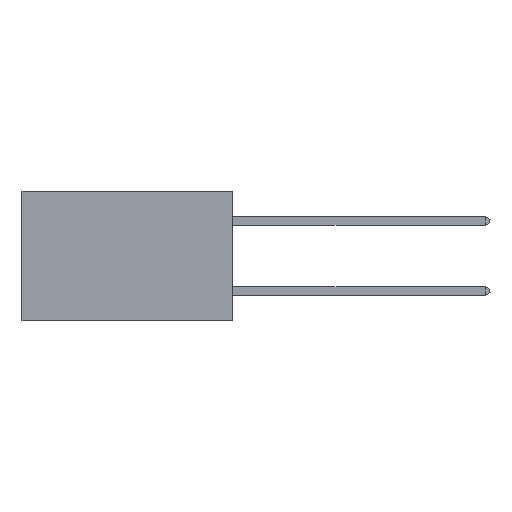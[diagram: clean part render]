
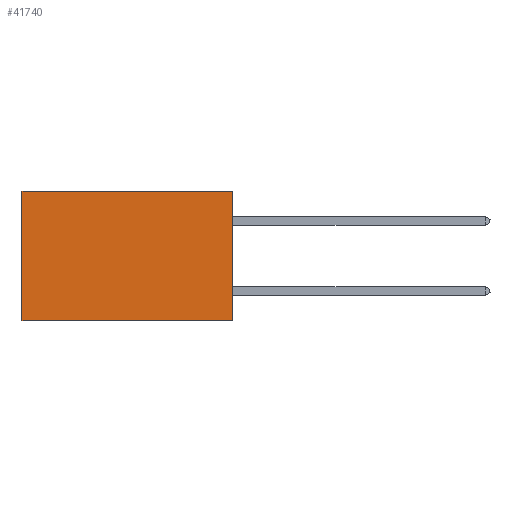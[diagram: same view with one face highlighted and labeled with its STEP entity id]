
A CAD part, left-side view. The second image highlights one B-rep face of the part: STEP entity #41740.
In plain terms, the highlighted planar face has unit normal (-1, 0, 0).
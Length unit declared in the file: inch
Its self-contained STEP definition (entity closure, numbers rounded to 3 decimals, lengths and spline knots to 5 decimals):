
#537 = CARTESIAN_POINT ( 'NONE',  ( 0.2875, 0., -0.37 ) ) ;
#599 = CARTESIAN_POINT ( 'NONE',  ( 0.2875, 0., 0. ) ) ;
#830 = CARTESIAN_POINT ( 'NONE',  ( 0.2875, 0.6, -0.37 ) ) ;
#4284 = VECTOR ( 'NONE', #30033, 39.37008 ) ;
#4651 = CARTESIAN_POINT ( 'NONE',  ( 0.2875, 0., 0. ) ) ;
#6736 = EDGE_LOOP ( 'NONE', ( #36808, #8428, #26859, #41243 ) ) ;
#8428 = ORIENTED_EDGE ( 'NONE', *, *, #11551, .F. ) ;
#8730 = CARTESIAN_POINT ( 'NONE',  ( 0.2875, 0., 0. ) ) ;
#10427 = CARTESIAN_POINT ( 'NONE',  ( 0.2875, 0.6, 0. ) ) ;
#11551 = EDGE_CURVE ( 'NONE', #14168, #26108, #36456, .T. ) ;
#12098 = DIRECTION ( 'NONE',  ( 0., 0., -1. ) ) ;
#13229 = CARTESIAN_POINT ( 'NONE',  ( 0.2875, 0., 0. ) ) ;
#14168 = VERTEX_POINT ( 'NONE', #537 ) ;
#17994 = VECTOR ( 'NONE', #19242, 39.37008 ) ;
#19242 = DIRECTION ( 'NONE',  ( 0., 1., 0. ) ) ;
#19360 = VECTOR ( 'NONE', #31343, 39.37008 ) ;
#21993 = PLANE ( 'NONE',  #40230 ) ;
#23264 = LINE ( 'NONE', #13229, #4284 ) ;
#25990 = VERTEX_POINT ( 'NONE', #10427 ) ;
#26108 = VERTEX_POINT ( 'NONE', #830 ) ;
#26772 = LINE ( 'NONE', #599, #19360 ) ;
#26859 = ORIENTED_EDGE ( 'NONE', *, *, #33230, .F. ) ;
#30033 = DIRECTION ( 'NONE',  ( 0., 0., -1. ) ) ;
#30135 = VECTOR ( 'NONE', #39481, 39.37008 ) ;
#31343 = DIRECTION ( 'NONE',  ( 0., 1., 0. ) ) ;
#31681 = EDGE_CURVE ( 'NONE', #25990, #26108, #35382, .T. ) ;
#33230 = EDGE_CURVE ( 'NONE', #37076, #14168, #23264, .T. ) ;
#35382 = LINE ( 'NONE', #39338, #30135 ) ;
#35407 = EDGE_CURVE ( 'NONE', #37076, #25990, #26772, .T. ) ;
#36456 = LINE ( 'NONE', #42908, #17994 ) ;
#36808 = ORIENTED_EDGE ( 'NONE', *, *, #31681, .T. ) ;
#37076 = VERTEX_POINT ( 'NONE', #4651 ) ;
#37758 = FACE_OUTER_BOUND ( 'NONE', #6736, .T. ) ;
#38581 = DIRECTION ( 'NONE',  ( 1., 0., 0. ) ) ;
#39338 = CARTESIAN_POINT ( 'NONE',  ( 0.2875, 0.6, 0. ) ) ;
#39481 = DIRECTION ( 'NONE',  ( 0., 0., -1. ) ) ;
#40230 = AXIS2_PLACEMENT_3D ( 'NONE', #8730, #38581, #12098 ) ;
#41243 = ORIENTED_EDGE ( 'NONE', *, *, #35407, .T. ) ;
#41740 = ADVANCED_FACE ( 'NONE', ( #37758 ), #21993, .F. ) ;
#42908 = CARTESIAN_POINT ( 'NONE',  ( 0.2875, 0., -0.37 ) ) ;
